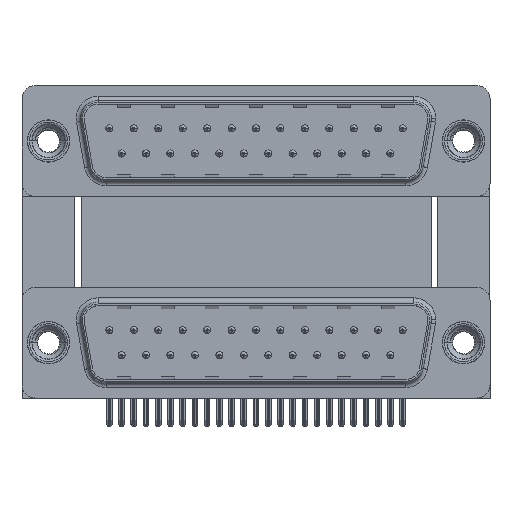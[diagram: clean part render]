
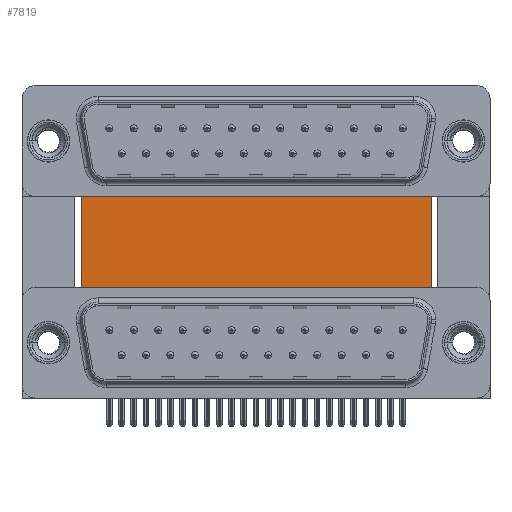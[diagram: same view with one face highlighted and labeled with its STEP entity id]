
A CAD part, top view. The second image highlights one B-rep face of the part: STEP entity #7819.
In plain terms, the highlighted planar face has unit normal (0, 0, 1).
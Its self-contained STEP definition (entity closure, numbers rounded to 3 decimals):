
#649 = DIRECTION ( 'NONE',  ( 0., -1., 0. ) ) ;
#875 = CARTESIAN_POINT ( 'NONE',  ( 43.43, 16.585, -12. ) ) ;
#2696 = DIRECTION ( 'NONE',  ( 1., 0., 0. ) ) ;
#2902 = LINE ( 'NONE', #31271, #29325 ) ;
#7819 = ADVANCED_FACE ( 'NONE', ( #24966 ), #16192, .F. ) ;
#9659 = DIRECTION ( 'NONE',  ( -1., 0., 0. ) ) ;
#10064 = DIRECTION ( 'NONE',  ( 0., -1., 0. ) ) ;
#10443 = VECTOR ( 'NONE', #2696, 1000. ) ;
#12319 = DIRECTION ( 'NONE',  ( 1., 0., 0. ) ) ;
#12721 = CARTESIAN_POINT ( 'NONE',  ( 3.79, -3.735, -12. ) ) ;
#13410 = VERTEX_POINT ( 'NONE', #31814 ) ;
#13568 = ORIENTED_EDGE ( 'NONE', *, *, #18816, .T. ) ;
#14961 = CARTESIAN_POINT ( 'NONE',  ( 3.79, 16.585, -12. ) ) ;
#15453 = VECTOR ( 'NONE', #12319, 1000. ) ;
#16001 = EDGE_CURVE ( 'NONE', #39765, #19471, #2902, .T. ) ;
#16192 = PLANE ( 'NONE',  #28792 ) ;
#16519 = CARTESIAN_POINT ( 'NONE',  ( 3.79, -3.735, -12. ) ) ;
#17894 = CARTESIAN_POINT ( 'NONE',  ( 3.79, 16.585, -12. ) ) ;
#18330 = ORIENTED_EDGE ( 'NONE', *, *, #16001, .T. ) ;
#18816 = EDGE_CURVE ( 'NONE', #19471, #18945, #31285, .T. ) ;
#18945 = VERTEX_POINT ( 'NONE', #22497 ) ;
#19471 = VERTEX_POINT ( 'NONE', #16519 ) ;
#22497 = CARTESIAN_POINT ( 'NONE',  ( 43.43, -3.735, -12. ) ) ;
#23836 = EDGE_CURVE ( 'NONE', #13410, #18945, #35561, .T. ) ;
#24778 = CARTESIAN_POINT ( 'NONE',  ( 3.79, 16.585, -12. ) ) ;
#24961 = VECTOR ( 'NONE', #10064, 1000. ) ;
#24966 = FACE_OUTER_BOUND ( 'NONE', #28274, .T. ) ;
#28032 = DIRECTION ( 'NONE',  ( 0., 0., -1. ) ) ;
#28274 = EDGE_LOOP ( 'NONE', ( #13568, #30569, #29641, #18330 ) ) ;
#28792 = AXIS2_PLACEMENT_3D ( 'NONE', #17894, #28032, #9659 ) ;
#29325 = VECTOR ( 'NONE', #649, 1000. ) ;
#29641 = ORIENTED_EDGE ( 'NONE', *, *, #31176, .F. ) ;
#30569 = ORIENTED_EDGE ( 'NONE', *, *, #23836, .F. ) ;
#31176 = EDGE_CURVE ( 'NONE', #39765, #13410, #40257, .T. ) ;
#31271 = CARTESIAN_POINT ( 'NONE',  ( 3.79, 16.585, -12. ) ) ;
#31285 = LINE ( 'NONE', #12721, #15453 ) ;
#31814 = CARTESIAN_POINT ( 'NONE',  ( 43.43, 16.585, -12. ) ) ;
#35561 = LINE ( 'NONE', #875, #24961 ) ;
#39765 = VERTEX_POINT ( 'NONE', #24778 ) ;
#40257 = LINE ( 'NONE', #14961, #10443 ) ;
